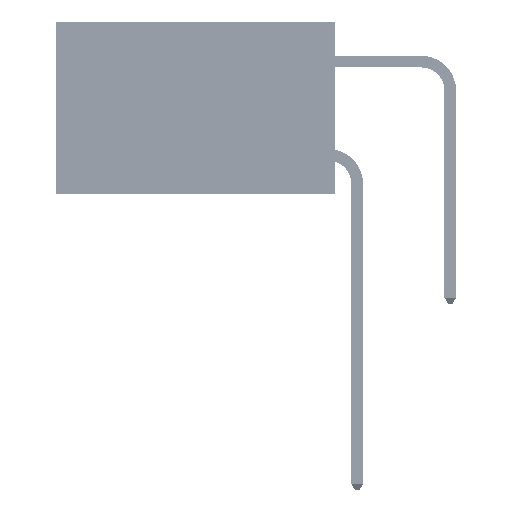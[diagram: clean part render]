
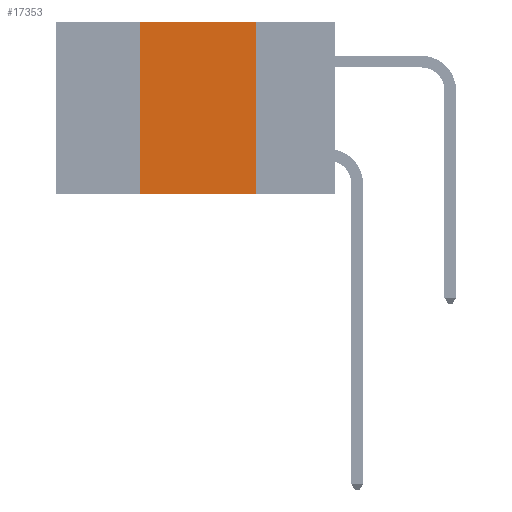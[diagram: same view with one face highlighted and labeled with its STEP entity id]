
A CAD part, left-side view. The second image highlights one B-rep face of the part: STEP entity #17353.
In plain terms, the highlighted planar face has unit normal (-1, 0, 0).
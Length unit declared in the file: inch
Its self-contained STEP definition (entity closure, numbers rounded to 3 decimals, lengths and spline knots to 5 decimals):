
#1091 = DIRECTION ( 'NONE',  ( 0., -1., 0. ) ) ;
#1280 = VECTOR ( 'NONE', #1091, 39.37008 ) ;
#8533 = LINE ( 'NONE', #35010, #1280 ) ;
#9832 = VERTEX_POINT ( 'NONE', #40690 ) ;
#13207 = VECTOR ( 'NONE', #14347, 39.37008 ) ;
#14017 = DIRECTION ( 'NONE',  ( 0., -1., 0. ) ) ;
#14347 = DIRECTION ( 'NONE',  ( 0., 0., 1. ) ) ;
#14838 = EDGE_LOOP ( 'NONE', ( #42796, #44853, #51447, #45901 ) ) ;
#17353 = ADVANCED_FACE ( 'NONE', ( #42245 ), #47269, .F. ) ;
#18055 = CARTESIAN_POINT ( 'NONE',  ( 0., 0.6, 0. ) ) ;
#18145 = CARTESIAN_POINT ( 'NONE',  ( 0., 0.6, 0. ) ) ;
#19429 = LINE ( 'NONE', #33189, #44333 ) ;
#23593 = LINE ( 'NONE', #18055, #25588 ) ;
#24360 = VERTEX_POINT ( 'NONE', #30830 ) ;
#25325 = DIRECTION ( 'NONE',  ( 0., 0., -1. ) ) ;
#25588 = VECTOR ( 'NONE', #14017, 39.37008 ) ;
#26397 = CARTESIAN_POINT ( 'NONE',  ( 0., 0.42, -0.37 ) ) ;
#26752 = DIRECTION ( 'NONE',  ( 1., 0., 0. ) ) ;
#26894 = EDGE_CURVE ( 'NONE', #24360, #28002, #23593, .T. ) ;
#28002 = VERTEX_POINT ( 'NONE', #28936 ) ;
#28936 = CARTESIAN_POINT ( 'NONE',  ( 0., 0.17, 0. ) ) ;
#30830 = CARTESIAN_POINT ( 'NONE',  ( 0., 0.42, 0. ) ) ;
#31866 = AXIS2_PLACEMENT_3D ( 'NONE', #18145, #26752, #48686 ) ;
#33189 = CARTESIAN_POINT ( 'NONE',  ( 0., 0.17, 0. ) ) ;
#33711 = EDGE_CURVE ( 'NONE', #35432, #9832, #8533, .T. ) ;
#35010 = CARTESIAN_POINT ( 'NONE',  ( 0., 0.6, -0.37 ) ) ;
#35384 = CARTESIAN_POINT ( 'NONE',  ( 0., 0.42, 0. ) ) ;
#35432 = VERTEX_POINT ( 'NONE', #26397 ) ;
#40690 = CARTESIAN_POINT ( 'NONE',  ( 0., 0.17, -0.37 ) ) ;
#42245 = FACE_OUTER_BOUND ( 'NONE', #14838, .T. ) ;
#42796 = ORIENTED_EDGE ( 'NONE', *, *, #49296, .F. ) ;
#44333 = VECTOR ( 'NONE', #25325, 39.37008 ) ;
#44853 = ORIENTED_EDGE ( 'NONE', *, *, #26894, .F. ) ;
#45901 = ORIENTED_EDGE ( 'NONE', *, *, #33711, .T. ) ;
#47269 = PLANE ( 'NONE',  #31866 ) ;
#48686 = DIRECTION ( 'NONE',  ( 0., 0., -1. ) ) ;
#49296 = EDGE_CURVE ( 'NONE', #28002, #9832, #19429, .T. ) ;
#51447 = ORIENTED_EDGE ( 'NONE', *, *, #51788, .F. ) ;
#51788 = EDGE_CURVE ( 'NONE', #35432, #24360, #53102, .T. ) ;
#53102 = LINE ( 'NONE', #35384, #13207 ) ;
